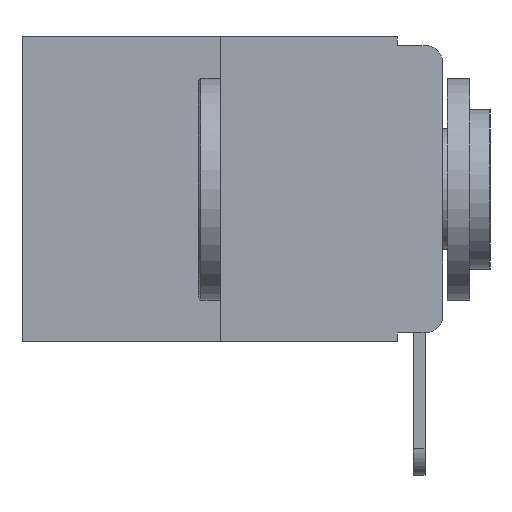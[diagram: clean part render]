
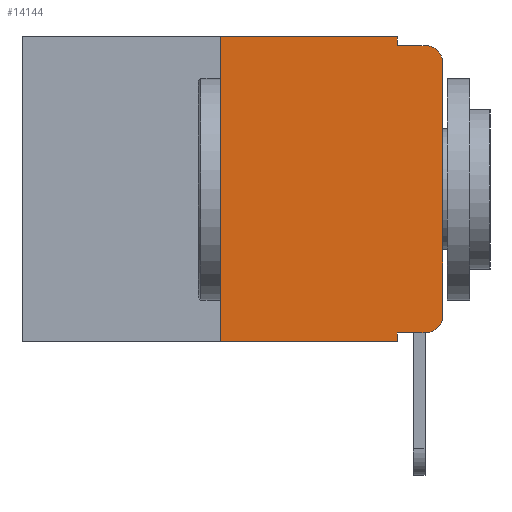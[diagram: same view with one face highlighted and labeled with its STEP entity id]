
A CAD part, left-side view. The second image highlights one B-rep face of the part: STEP entity #14144.
In plain terms, the highlighted planar face has unit normal (-1, 0, 0).
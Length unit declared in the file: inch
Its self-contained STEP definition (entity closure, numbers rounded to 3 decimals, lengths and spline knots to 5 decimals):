
#331 = ORIENTED_EDGE ( 'NONE', *, *, #13511, .T. ) ;
#670 = VERTEX_POINT ( 'NONE', #16211 ) ;
#982 = DIRECTION ( 'NONE',  ( -1., 0., 0. ) ) ;
#1037 = ORIENTED_EDGE ( 'NONE', *, *, #16765, .F. ) ;
#1434 = VERTEX_POINT ( 'NONE', #16918 ) ;
#2049 = CARTESIAN_POINT ( 'NONE',  ( 0., 0.051, 0. ) ) ;
#2188 = VERTEX_POINT ( 'NONE', #8853 ) ;
#2271 = CARTESIAN_POINT ( 'NONE',  ( 0., 0.051, -0.333 ) ) ;
#2338 = DIRECTION ( 'NONE',  ( 0., -1., 0. ) ) ;
#2397 = VERTEX_POINT ( 'NONE', #16303 ) ;
#2407 = CARTESIAN_POINT ( 'NONE',  ( 0., 0.051, -0.01 ) ) ;
#2558 = DIRECTION ( 'NONE',  ( 0., 0., 1. ) ) ;
#2614 = ORIENTED_EDGE ( 'NONE', *, *, #9135, .T. ) ;
#2913 = VECTOR ( 'NONE', #15048, 39.37008 ) ;
#3007 = VERTEX_POINT ( 'NONE', #11189 ) ;
#3022 = VECTOR ( 'NONE', #13919, 39.37008 ) ;
#3217 = LINE ( 'NONE', #4043, #3022 ) ;
#3240 = AXIS2_PLACEMENT_3D ( 'NONE', #14840, #10428, #14715 ) ;
#3351 = ORIENTED_EDGE ( 'NONE', *, *, #14628, .T. ) ;
#3607 = EDGE_LOOP ( 'NONE', ( #3351, #2614, #1037, #12794, #17722, #7814, #6714, #16245, #14252, #331 ) ) ;
#3613 = LINE ( 'NONE', #2407, #11318 ) ;
#3920 = CARTESIAN_POINT ( 'NONE',  ( 0., 0.25, 0. ) ) ;
#4043 = CARTESIAN_POINT ( 'NONE',  ( 0., 0.473, 0. ) ) ;
#5175 = CARTESIAN_POINT ( 'NONE',  ( 0., 0., -0.03 ) ) ;
#5840 = AXIS2_PLACEMENT_3D ( 'NONE', #14953, #982, #9290 ) ;
#5842 = LINE ( 'NONE', #3920, #11359 ) ;
#6030 = LINE ( 'NONE', #2271, #7116 ) ;
#6156 = VERTEX_POINT ( 'NONE', #16592 ) ;
#6160 = CIRCLE ( 'NONE', #5840, 0.02 ) ;
#6186 = DIRECTION ( 'NONE',  ( 0., 0., -1. ) ) ;
#6663 = LINE ( 'NONE', #12360, #2913 ) ;
#6714 = ORIENTED_EDGE ( 'NONE', *, *, #12280, .T. ) ;
#6867 = DIRECTION ( 'NONE',  ( 0., 0., -1. ) ) ;
#6868 = DIRECTION ( 'NONE',  ( 0., 0., -1. ) ) ;
#7116 = VECTOR ( 'NONE', #2338, 39.37008 ) ;
#7666 = EDGE_CURVE ( 'NONE', #13913, #16655, #3217, .T. ) ;
#7814 = ORIENTED_EDGE ( 'NONE', *, *, #10121, .F. ) ;
#8057 = CARTESIAN_POINT ( 'NONE',  ( 0., 0.25, -0.343 ) ) ;
#8853 = CARTESIAN_POINT ( 'NONE',  ( 0., 0.02, -0.333 ) ) ;
#9133 = CIRCLE ( 'NONE', #10421, 0.02 ) ;
#9135 = EDGE_CURVE ( 'NONE', #15927, #3007, #9133, .T. ) ;
#9160 = DIRECTION ( 'NONE',  ( 0., 0., 1. ) ) ;
#9290 = DIRECTION ( 'NONE',  ( 0., 0., -1. ) ) ;
#9365 = LINE ( 'NONE', #2049, #10468 ) ;
#9458 = VECTOR ( 'NONE', #6867, 39.37008 ) ;
#9480 = DIRECTION ( 'NONE',  ( -1., 0., 0. ) ) ;
#10121 = EDGE_CURVE ( 'NONE', #17265, #13913, #5842, .T. ) ;
#10421 = AXIS2_PLACEMENT_3D ( 'NONE', #15197, #9480, #6868 ) ;
#10428 = DIRECTION ( 'NONE',  ( 1., 0., 0. ) ) ;
#10468 = VECTOR ( 'NONE', #6186, 39.37008 ) ;
#10523 = EDGE_CURVE ( 'NONE', #16655, #1434, #9365, .T. ) ;
#10743 = DIRECTION ( 'NONE',  ( 0., -1., 0. ) ) ;
#10767 = EDGE_CURVE ( 'NONE', #2397, #2188, #6030, .T. ) ;
#11189 = CARTESIAN_POINT ( 'NONE',  ( 0., 0.02, -0.01 ) ) ;
#11318 = VECTOR ( 'NONE', #10743, 39.37008 ) ;
#11359 = VECTOR ( 'NONE', #2558, 39.37008 ) ;
#12117 = LINE ( 'NONE', #15255, #9458 ) ;
#12280 = EDGE_CURVE ( 'NONE', #17265, #6156, #6663, .T. ) ;
#12360 = CARTESIAN_POINT ( 'NONE',  ( 0., 0.473, -0.343 ) ) ;
#12794 = ORIENTED_EDGE ( 'NONE', *, *, #10523, .F. ) ;
#13187 = PLANE ( 'NONE',  #3240 ) ;
#13511 = EDGE_CURVE ( 'NONE', #2188, #670, #6160, .T. ) ;
#13626 = EDGE_CURVE ( 'NONE', #2397, #6156, #12117, .T. ) ;
#13913 = VERTEX_POINT ( 'NONE', #14233 ) ;
#13919 = DIRECTION ( 'NONE',  ( 0., -1., 0. ) ) ;
#14144 = ADVANCED_FACE ( 'NONE', ( #17364 ), #13187, .F. ) ;
#14233 = CARTESIAN_POINT ( 'NONE',  ( 0., 0.25, 0. ) ) ;
#14252 = ORIENTED_EDGE ( 'NONE', *, *, #10767, .T. ) ;
#14253 = VECTOR ( 'NONE', #9160, 39.37008 ) ;
#14628 = EDGE_CURVE ( 'NONE', #670, #15927, #14688, .T. ) ;
#14688 = LINE ( 'NONE', #17587, #14253 ) ;
#14715 = DIRECTION ( 'NONE',  ( 0., 0., -1. ) ) ;
#14840 = CARTESIAN_POINT ( 'NONE',  ( 0., 0.473, 0. ) ) ;
#14953 = CARTESIAN_POINT ( 'NONE',  ( 0., 0.02, -0.313 ) ) ;
#15048 = DIRECTION ( 'NONE',  ( 0., -1., 0. ) ) ;
#15197 = CARTESIAN_POINT ( 'NONE',  ( 0., 0.02, -0.03 ) ) ;
#15255 = CARTESIAN_POINT ( 'NONE',  ( 0., 0.051, 0. ) ) ;
#15927 = VERTEX_POINT ( 'NONE', #5175 ) ;
#16030 = CARTESIAN_POINT ( 'NONE',  ( 0., 0.051, 0. ) ) ;
#16211 = CARTESIAN_POINT ( 'NONE',  ( 0., 0., -0.313 ) ) ;
#16245 = ORIENTED_EDGE ( 'NONE', *, *, #13626, .F. ) ;
#16303 = CARTESIAN_POINT ( 'NONE',  ( 0., 0.051, -0.333 ) ) ;
#16592 = CARTESIAN_POINT ( 'NONE',  ( 0., 0.051, -0.343 ) ) ;
#16655 = VERTEX_POINT ( 'NONE', #16030 ) ;
#16765 = EDGE_CURVE ( 'NONE', #1434, #3007, #3613, .T. ) ;
#16918 = CARTESIAN_POINT ( 'NONE',  ( 0., 0.051, -0.01 ) ) ;
#17265 = VERTEX_POINT ( 'NONE', #8057 ) ;
#17364 = FACE_OUTER_BOUND ( 'NONE', #3607, .T. ) ;
#17587 = CARTESIAN_POINT ( 'NONE',  ( 0., 0., 0. ) ) ;
#17722 = ORIENTED_EDGE ( 'NONE', *, *, #7666, .F. ) ;
